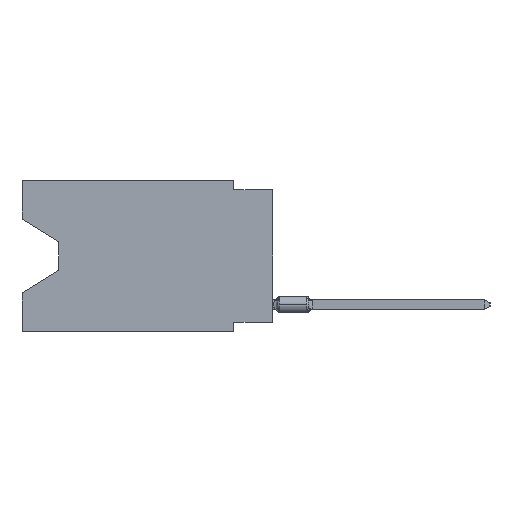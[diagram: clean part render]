
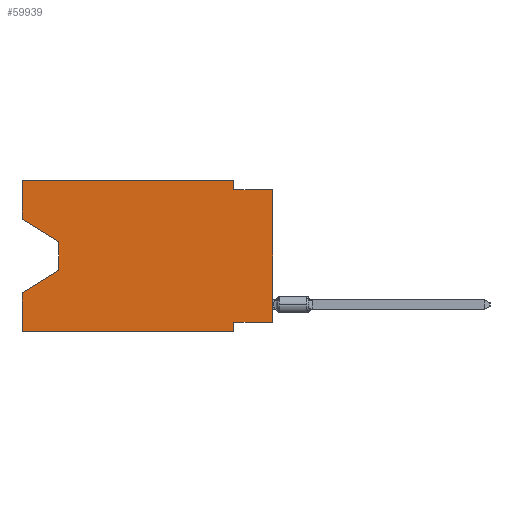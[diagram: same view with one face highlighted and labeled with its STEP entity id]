
A CAD part, left-side view. The second image highlights one B-rep face of the part: STEP entity #59939.
In plain terms, the highlighted planar face has unit normal (-1, 0, 0).
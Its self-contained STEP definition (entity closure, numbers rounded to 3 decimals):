
#188 = VECTOR ( 'NONE', #40477, 1000. ) ;
#1706 = ORIENTED_EDGE ( 'NONE', *, *, #12107, .F. ) ;
#2247 = VERTEX_POINT ( 'NONE', #80851 ) ;
#2671 = DIRECTION ( 'NONE',  ( 0., 0., -1. ) ) ;
#6421 = VECTOR ( 'NONE', #63292, 1000. ) ;
#7845 = DIRECTION ( 'NONE',  ( 0., 0., 1. ) ) ;
#8361 = ORIENTED_EDGE ( 'NONE', *, *, #54646, .T. ) ;
#9041 = VECTOR ( 'NONE', #55729, 1000. ) ;
#9072 = CARTESIAN_POINT ( 'NONE',  ( 0., 16.383, 0. ) ) ;
#10070 = VERTEX_POINT ( 'NONE', #15965 ) ;
#10617 = LINE ( 'NONE', #37779, #17746 ) ;
#12107 = EDGE_CURVE ( 'NONE', #49695, #44846, #67159, .T. ) ;
#13752 = CARTESIAN_POINT ( 'NONE',  ( 0., 2.54, 0. ) ) ;
#14056 = EDGE_CURVE ( 'NONE', #23430, #2247, #43761, .T. ) ;
#14580 = LINE ( 'NONE', #13752, #188 ) ;
#15812 = ORIENTED_EDGE ( 'NONE', *, *, #64533, .T. ) ;
#15965 = CARTESIAN_POINT ( 'NONE',  ( 0., 2.54, -9.906 ) ) ;
#16317 = LINE ( 'NONE', #66440, #23777 ) ;
#17658 = VERTEX_POINT ( 'NONE', #80447 ) ;
#17746 = VECTOR ( 'NONE', #56480, 1000. ) ;
#17940 = EDGE_CURVE ( 'NONE', #71268, #81943, #70309, .T. ) ;
#18514 = VERTEX_POINT ( 'NONE', #75115 ) ;
#18583 = DIRECTION ( 'NONE',  ( 0., -0.855, -0.519 ) ) ;
#20122 = CARTESIAN_POINT ( 'NONE',  ( 0., 16.383, 0. ) ) ;
#20942 = VECTOR ( 'NONE', #60604, 1000. ) ;
#22875 = EDGE_CURVE ( 'NONE', #37316, #40480, #30467, .T. ) ;
#23076 = VERTEX_POINT ( 'NONE', #52497 ) ;
#23430 = VERTEX_POINT ( 'NONE', #27642 ) ;
#23777 = VECTOR ( 'NONE', #7845, 1000. ) ;
#24633 = CARTESIAN_POINT ( 'NONE',  ( 0., 16.383, 0. ) ) ;
#24876 = VECTOR ( 'NONE', #18583, 1000. ) ;
#25230 = VECTOR ( 'NONE', #73969, 1000. ) ;
#26270 = EDGE_CURVE ( 'NONE', #17658, #18514, #70674, .T. ) ;
#27345 = FACE_OUTER_BOUND ( 'NONE', #69454, .T. ) ;
#27642 = CARTESIAN_POINT ( 'NONE',  ( 0., 16.383, -9.906 ) ) ;
#30467 = LINE ( 'NONE', #50844, #24876 ) ;
#31306 = VECTOR ( 'NONE', #52834, 1000. ) ;
#32289 = ORIENTED_EDGE ( 'NONE', *, *, #41133, .T. ) ;
#34261 = LINE ( 'NONE', #41061, #20942 ) ;
#37316 = VERTEX_POINT ( 'NONE', #50596 ) ;
#37779 = CARTESIAN_POINT ( 'NONE',  ( 0., 2.54, -9.906 ) ) ;
#37996 = VECTOR ( 'NONE', #65160, 1000. ) ;
#39228 = DIRECTION ( 'NONE',  ( 0., 1., 0. ) ) ;
#40477 = DIRECTION ( 'NONE',  ( 0., 0., -1. ) ) ;
#40480 = VERTEX_POINT ( 'NONE', #73079 ) ;
#41061 = CARTESIAN_POINT ( 'NONE',  ( 0., 13.97, -5.893 ) ) ;
#41133 = EDGE_CURVE ( 'NONE', #40480, #23076, #59350, .T. ) ;
#41344 = PLANE ( 'NONE',  #63477 ) ;
#42567 = CARTESIAN_POINT ( 'NONE',  ( 0., 16.383, -9.906 ) ) ;
#43658 = VECTOR ( 'NONE', #52967, 1000. ) ;
#43761 = LINE ( 'NONE', #24633, #6421 ) ;
#44846 = VERTEX_POINT ( 'NONE', #78341 ) ;
#47631 = CARTESIAN_POINT ( 'NONE',  ( 0., 16.383, 0. ) ) ;
#49695 = VERTEX_POINT ( 'NONE', #60927 ) ;
#50203 = LINE ( 'NONE', #42567, #9041 ) ;
#50596 = CARTESIAN_POINT ( 'NONE',  ( 0., 16.383, -2.546 ) ) ;
#50844 = CARTESIAN_POINT ( 'NONE',  ( 0., 16.383, -2.546 ) ) ;
#51312 = ORIENTED_EDGE ( 'NONE', *, *, #62341, .F. ) ;
#52497 = CARTESIAN_POINT ( 'NONE',  ( 0., 13.97, -5.893 ) ) ;
#52834 = DIRECTION ( 'NONE',  ( 0., -1., 0. ) ) ;
#52967 = DIRECTION ( 'NONE',  ( 0., 0., -1. ) ) ;
#54646 = EDGE_CURVE ( 'NONE', #23076, #2247, #34261, .T. ) ;
#55729 = DIRECTION ( 'NONE',  ( 0., -1., 0. ) ) ;
#56480 = DIRECTION ( 'NONE',  ( 0., 0., -1. ) ) ;
#57975 = CARTESIAN_POINT ( 'NONE',  ( 0., 0., -0.635 ) ) ;
#58842 = ORIENTED_EDGE ( 'NONE', *, *, #17940, .F. ) ;
#58952 = ORIENTED_EDGE ( 'NONE', *, *, #70903, .F. ) ;
#59350 = LINE ( 'NONE', #66957, #43658 ) ;
#59939 = ADVANCED_FACE ( 'NONE', ( #27345 ), #41344, .F. ) ;
#60604 = DIRECTION ( 'NONE',  ( 0., 0.855, -0.519 ) ) ;
#60873 = DIRECTION ( 'NONE',  ( 1., 0., 0. ) ) ;
#60927 = CARTESIAN_POINT ( 'NONE',  ( 0., 16.383, 0. ) ) ;
#62341 = EDGE_CURVE ( 'NONE', #37316, #49695, #70289, .T. ) ;
#63292 = DIRECTION ( 'NONE',  ( 0., 0., 1. ) ) ;
#63477 = AXIS2_PLACEMENT_3D ( 'NONE', #9072, #60873, #2671 ) ;
#64533 = EDGE_CURVE ( 'NONE', #23430, #10070, #50203, .T. ) ;
#65160 = DIRECTION ( 'NONE',  ( 0., 0., 1. ) ) ;
#66239 = VECTOR ( 'NONE', #39228, 1000. ) ;
#66440 = CARTESIAN_POINT ( 'NONE',  ( 0., 0., 0. ) ) ;
#66599 = CARTESIAN_POINT ( 'NONE',  ( 0., 2.54, -0.635 ) ) ;
#66957 = CARTESIAN_POINT ( 'NONE',  ( 0., 13.97, -4.013 ) ) ;
#67159 = LINE ( 'NONE', #47631, #25230 ) ;
#68738 = ORIENTED_EDGE ( 'NONE', *, *, #76071, .T. ) ;
#69454 = EDGE_LOOP ( 'NONE', ( #72343, #32289, #8361, #74916, #15812, #72959, #81220, #68738, #58842, #58952, #1706, #51312 ) ) ;
#70095 = EDGE_CURVE ( 'NONE', #18514, #10070, #10617, .T. ) ;
#70289 = LINE ( 'NONE', #20122, #37996 ) ;
#70309 = LINE ( 'NONE', #57975, #31306 ) ;
#70674 = LINE ( 'NONE', #77070, #66239 ) ;
#70903 = EDGE_CURVE ( 'NONE', #44846, #71268, #14580, .T. ) ;
#71268 = VERTEX_POINT ( 'NONE', #66599 ) ;
#72343 = ORIENTED_EDGE ( 'NONE', *, *, #22875, .T. ) ;
#72959 = ORIENTED_EDGE ( 'NONE', *, *, #70095, .F. ) ;
#73079 = CARTESIAN_POINT ( 'NONE',  ( 0., 13.97, -4.013 ) ) ;
#73969 = DIRECTION ( 'NONE',  ( 0., -1., 0. ) ) ;
#74916 = ORIENTED_EDGE ( 'NONE', *, *, #14056, .F. ) ;
#74977 = CARTESIAN_POINT ( 'NONE',  ( 0., 0., -0.635 ) ) ;
#75115 = CARTESIAN_POINT ( 'NONE',  ( 0., 2.54, -9.271 ) ) ;
#76071 = EDGE_CURVE ( 'NONE', #17658, #81943, #16317, .T. ) ;
#77070 = CARTESIAN_POINT ( 'NONE',  ( 0., 0., -9.271 ) ) ;
#78341 = CARTESIAN_POINT ( 'NONE',  ( 0., 2.54, 0. ) ) ;
#80447 = CARTESIAN_POINT ( 'NONE',  ( 0., 0., -9.271 ) ) ;
#80851 = CARTESIAN_POINT ( 'NONE',  ( 0., 16.383, -7.36 ) ) ;
#81220 = ORIENTED_EDGE ( 'NONE', *, *, #26270, .F. ) ;
#81943 = VERTEX_POINT ( 'NONE', #74977 ) ;
